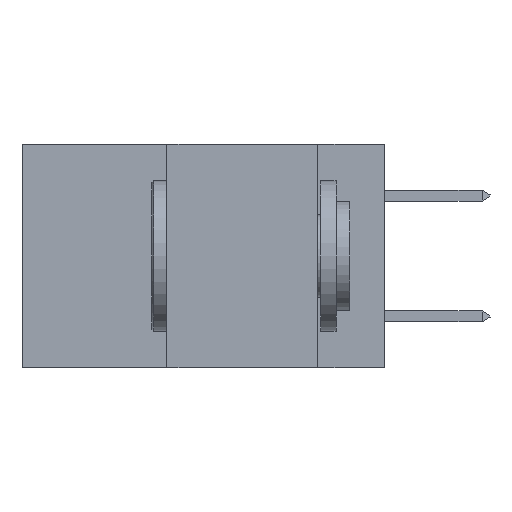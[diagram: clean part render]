
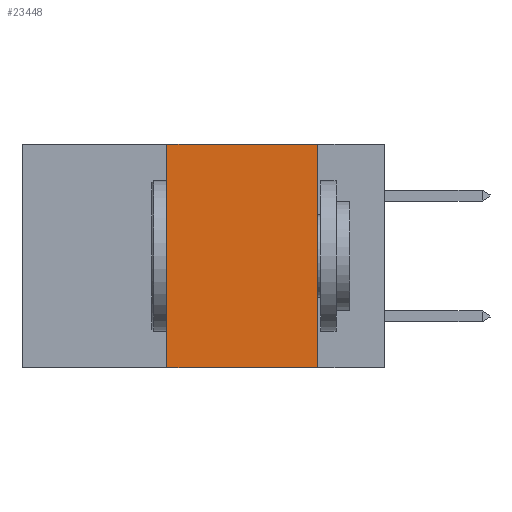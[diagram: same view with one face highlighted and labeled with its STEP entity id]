
A CAD part, left-side view. The second image highlights one B-rep face of the part: STEP entity #23448.
In plain terms, the highlighted planar face has unit normal (-1, 0, 0).
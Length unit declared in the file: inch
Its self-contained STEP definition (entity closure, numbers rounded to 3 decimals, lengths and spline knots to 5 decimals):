
#2357 = ORIENTED_EDGE ( 'NONE', *, *, #30739, .F. ) ;
#4148 = DIRECTION ( 'NONE',  ( 0., 0., -1. ) ) ;
#4972 = CARTESIAN_POINT ( 'NONE',  ( 0., 0.6, 0. ) ) ;
#5019 = AXIS2_PLACEMENT_3D ( 'NONE', #35067, #21008, #4148 ) ;
#5069 = CARTESIAN_POINT ( 'NONE',  ( 0., 0.36, 0. ) ) ;
#5470 = LINE ( 'NONE', #13369, #19549 ) ;
#8523 = ORIENTED_EDGE ( 'NONE', *, *, #35679, .F. ) ;
#10037 = EDGE_LOOP ( 'NONE', ( #8523, #23507, #2357, #16876 ) ) ;
#11425 = VERTEX_POINT ( 'NONE', #35794 ) ;
#12658 = VECTOR ( 'NONE', #33798, 39.37008 ) ;
#12894 = VERTEX_POINT ( 'NONE', #28540 ) ;
#13035 = VECTOR ( 'NONE', #15090, 39.37008 ) ;
#13369 = CARTESIAN_POINT ( 'NONE',  ( 0., 0.11, 0. ) ) ;
#13496 = DIRECTION ( 'NONE',  ( 0., 0., -1. ) ) ;
#14451 = VERTEX_POINT ( 'NONE', #20498 ) ;
#14824 = CARTESIAN_POINT ( 'NONE',  ( 0., 0.36, 0. ) ) ;
#14964 = FACE_OUTER_BOUND ( 'NONE', #10037, .T. ) ;
#15090 = DIRECTION ( 'NONE',  ( 0., -1., 0. ) ) ;
#16122 = VECTOR ( 'NONE', #30369, 39.37008 ) ;
#16876 = ORIENTED_EDGE ( 'NONE', *, *, #31431, .T. ) ;
#18171 = PLANE ( 'NONE',  #5019 ) ;
#19549 = VECTOR ( 'NONE', #13496, 39.37008 ) ;
#20149 = LINE ( 'NONE', #5069, #12658 ) ;
#20498 = CARTESIAN_POINT ( 'NONE',  ( 0., 0.36, -0.37 ) ) ;
#21008 = DIRECTION ( 'NONE',  ( 1., 0., 0. ) ) ;
#23448 = ADVANCED_FACE ( 'NONE', ( #14964 ), #18171, .F. ) ;
#23507 = ORIENTED_EDGE ( 'NONE', *, *, #25846, .F. ) ;
#23651 = LINE ( 'NONE', #4972, #16122 ) ;
#25846 = EDGE_CURVE ( 'NONE', #35999, #11425, #23651, .T. ) ;
#28078 = LINE ( 'NONE', #34835, #13035 ) ;
#28540 = CARTESIAN_POINT ( 'NONE',  ( 0., 0.11, -0.37 ) ) ;
#30369 = DIRECTION ( 'NONE',  ( 0., -1., 0. ) ) ;
#30739 = EDGE_CURVE ( 'NONE', #14451, #35999, #20149, .T. ) ;
#31431 = EDGE_CURVE ( 'NONE', #14451, #12894, #28078, .T. ) ;
#33798 = DIRECTION ( 'NONE',  ( 0., 0., 1. ) ) ;
#34835 = CARTESIAN_POINT ( 'NONE',  ( 0., 0.6, -0.37 ) ) ;
#35067 = CARTESIAN_POINT ( 'NONE',  ( 0., 0.6, 0. ) ) ;
#35679 = EDGE_CURVE ( 'NONE', #11425, #12894, #5470, .T. ) ;
#35794 = CARTESIAN_POINT ( 'NONE',  ( 0., 0.11, 0. ) ) ;
#35999 = VERTEX_POINT ( 'NONE', #14824 ) ;
